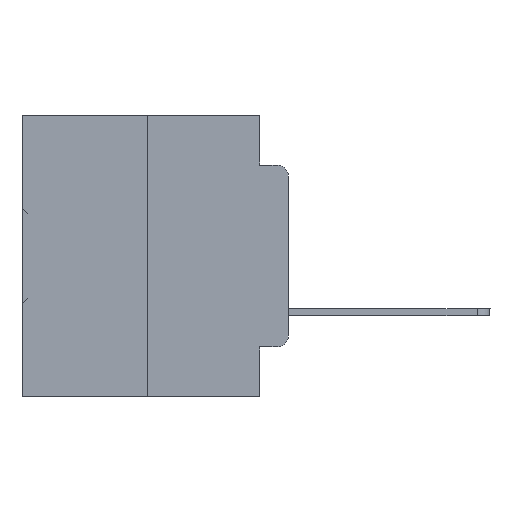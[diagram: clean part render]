
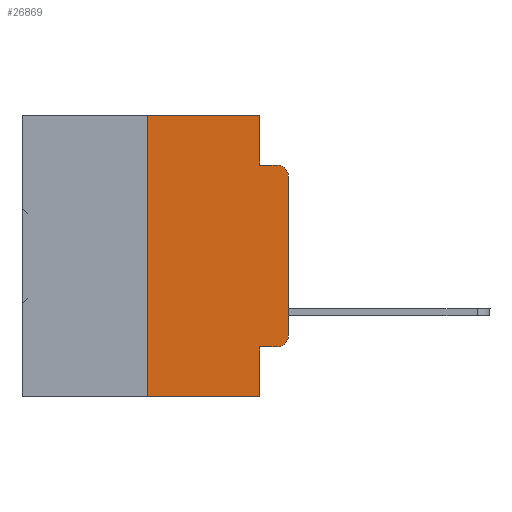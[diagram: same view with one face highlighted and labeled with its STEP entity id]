
A CAD part, left-side view. The second image highlights one B-rep face of the part: STEP entity #26869.
In plain terms, the highlighted planar face has unit normal (-1, 0, 0).
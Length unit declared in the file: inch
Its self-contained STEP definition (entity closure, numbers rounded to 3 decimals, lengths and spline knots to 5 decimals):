
#126 = VERTEX_POINT ( 'NONE', #30099 ) ;
#490 = LINE ( 'NONE', #19398, #20728 ) ;
#538 = ORIENTED_EDGE ( 'NONE', *, *, #15518, .T. ) ;
#1044 = VERTEX_POINT ( 'NONE', #1634 ) ;
#1201 = CARTESIAN_POINT ( 'NONE',  ( 0., 0.473, 0. ) ) ;
#1383 = VECTOR ( 'NONE', #17921, 39.37008 ) ;
#1459 = EDGE_CURVE ( 'NONE', #26376, #28990, #25783, .T. ) ;
#1634 = CARTESIAN_POINT ( 'NONE',  ( 0., 0.051, -0.5 ) ) ;
#2122 = ORIENTED_EDGE ( 'NONE', *, *, #19905, .F. ) ;
#2358 = EDGE_CURVE ( 'NONE', #27264, #26376, #7809, .T. ) ;
#2531 = DIRECTION ( 'NONE',  ( 0., 0., -1. ) ) ;
#3385 = CARTESIAN_POINT ( 'NONE',  ( 0., 0.051, -0.4115 ) ) ;
#4069 = VECTOR ( 'NONE', #15227, 39.37008 ) ;
#5417 = ORIENTED_EDGE ( 'NONE', *, *, #25851, .T. ) ;
#5433 = CARTESIAN_POINT ( 'NONE',  ( 0., 0.02, -0.4115 ) ) ;
#5965 = EDGE_CURVE ( 'NONE', #28134, #1044, #12391, .T. ) ;
#6599 = VERTEX_POINT ( 'NONE', #24161 ) ;
#6782 = DIRECTION ( 'NONE',  ( 0., -1., 0. ) ) ;
#6869 = VERTEX_POINT ( 'NONE', #23663 ) ;
#7082 = DIRECTION ( 'NONE',  ( 0., 0., -1. ) ) ;
#7211 = CARTESIAN_POINT ( 'NONE',  ( 0., 0.473, -0.5 ) ) ;
#7809 = CIRCLE ( 'NONE', #18820, 0.02 ) ;
#7995 = CARTESIAN_POINT ( 'NONE',  ( 0., 0., -0.3915 ) ) ;
#8035 = CARTESIAN_POINT ( 'NONE',  ( 0., 0.25, -0.5 ) ) ;
#8960 = DIRECTION ( 'NONE',  ( 0., 0., -1. ) ) ;
#9674 = CARTESIAN_POINT ( 'NONE',  ( 0., 0.051, 0. ) ) ;
#9696 = CARTESIAN_POINT ( 'NONE',  ( 0., 0.051, -0.4115 ) ) ;
#9814 = LINE ( 'NONE', #20336, #25372 ) ;
#10351 = LINE ( 'NONE', #22161, #12991 ) ;
#10411 = PLANE ( 'NONE',  #27936 ) ;
#10488 = LINE ( 'NONE', #18305, #18706 ) ;
#10786 = EDGE_LOOP ( 'NONE', ( #19140, #538, #18006, #33242, #21873, #2122, #30700, #25112, #5417, #28269 ) ) ;
#10952 = VERTEX_POINT ( 'NONE', #8035 ) ;
#12114 = LINE ( 'NONE', #7211, #1383 ) ;
#12391 = LINE ( 'NONE', #9674, #32156 ) ;
#12475 = DIRECTION ( 'NONE',  ( -1., 0., 0. ) ) ;
#12529 = VERTEX_POINT ( 'NONE', #23662 ) ;
#12991 = VECTOR ( 'NONE', #30169, 39.37008 ) ;
#13649 = AXIS2_PLACEMENT_3D ( 'NONE', #26289, #12475, #15550 ) ;
#15193 = VECTOR ( 'NONE', #6782, 39.37008 ) ;
#15227 = DIRECTION ( 'NONE',  ( 0., 0., 1. ) ) ;
#15518 = EDGE_CURVE ( 'NONE', #28990, #6869, #16547, .T. ) ;
#15550 = DIRECTION ( 'NONE',  ( 0., 0., -1. ) ) ;
#16495 = DIRECTION ( 'NONE',  ( 0., 0., 1. ) ) ;
#16547 = CIRCLE ( 'NONE', #13649, 0.02 ) ;
#17921 = DIRECTION ( 'NONE',  ( 0., -1., 0. ) ) ;
#18006 = ORIENTED_EDGE ( 'NONE', *, *, #27863, .F. ) ;
#18305 = CARTESIAN_POINT ( 'NONE',  ( 0., 0.051, -0.0885 ) ) ;
#18568 = LINE ( 'NONE', #9696, #15193 ) ;
#18706 = VECTOR ( 'NONE', #20845, 39.37008 ) ;
#18820 = AXIS2_PLACEMENT_3D ( 'NONE', #24178, #35277, #2531 ) ;
#19140 = ORIENTED_EDGE ( 'NONE', *, *, #1459, .T. ) ;
#19398 = CARTESIAN_POINT ( 'NONE',  ( 0., 0.25, 0. ) ) ;
#19905 = EDGE_CURVE ( 'NONE', #10952, #126, #490, .T. ) ;
#20336 = CARTESIAN_POINT ( 'NONE',  ( 0., 0.051, 0. ) ) ;
#20728 = VECTOR ( 'NONE', #16495, 39.37008 ) ;
#20845 = DIRECTION ( 'NONE',  ( 0., -1., 0. ) ) ;
#21873 = ORIENTED_EDGE ( 'NONE', *, *, #29247, .F. ) ;
#22161 = CARTESIAN_POINT ( 'NONE',  ( 0., 0.473, 0. ) ) ;
#22381 = CARTESIAN_POINT ( 'NONE',  ( 0., 0., -0.1085 ) ) ;
#23033 = DIRECTION ( 'NONE',  ( 1., 0., 0. ) ) ;
#23662 = CARTESIAN_POINT ( 'NONE',  ( 0., 0.051, 0. ) ) ;
#23663 = CARTESIAN_POINT ( 'NONE',  ( 0., 0.02, -0.0885 ) ) ;
#24161 = CARTESIAN_POINT ( 'NONE',  ( 0., 0.051, -0.0885 ) ) ;
#24178 = CARTESIAN_POINT ( 'NONE',  ( 0., 0.02, -0.3915 ) ) ;
#25112 = ORIENTED_EDGE ( 'NONE', *, *, #5965, .F. ) ;
#25372 = VECTOR ( 'NONE', #7082, 39.37008 ) ;
#25783 = LINE ( 'NONE', #31790, #4069 ) ;
#25851 = EDGE_CURVE ( 'NONE', #28134, #27264, #18568, .T. ) ;
#26289 = CARTESIAN_POINT ( 'NONE',  ( 0., 0.02, -0.1085 ) ) ;
#26376 = VERTEX_POINT ( 'NONE', #7995 ) ;
#26869 = ADVANCED_FACE ( 'NONE', ( #31764 ), #10411, .F. ) ;
#27264 = VERTEX_POINT ( 'NONE', #5433 ) ;
#27863 = EDGE_CURVE ( 'NONE', #6599, #6869, #10488, .T. ) ;
#27936 = AXIS2_PLACEMENT_3D ( 'NONE', #1201, #23033, #32602 ) ;
#28134 = VERTEX_POINT ( 'NONE', #3385 ) ;
#28269 = ORIENTED_EDGE ( 'NONE', *, *, #2358, .T. ) ;
#28990 = VERTEX_POINT ( 'NONE', #22381 ) ;
#29247 = EDGE_CURVE ( 'NONE', #126, #12529, #10351, .T. ) ;
#30099 = CARTESIAN_POINT ( 'NONE',  ( 0., 0.25, 0. ) ) ;
#30169 = DIRECTION ( 'NONE',  ( 0., -1., 0. ) ) ;
#30700 = ORIENTED_EDGE ( 'NONE', *, *, #31389, .T. ) ;
#31389 = EDGE_CURVE ( 'NONE', #10952, #1044, #12114, .T. ) ;
#31764 = FACE_OUTER_BOUND ( 'NONE', #10786, .T. ) ;
#31790 = CARTESIAN_POINT ( 'NONE',  ( 0., 0., 0. ) ) ;
#32156 = VECTOR ( 'NONE', #8960, 39.37008 ) ;
#32602 = DIRECTION ( 'NONE',  ( 0., 0., -1. ) ) ;
#33242 = ORIENTED_EDGE ( 'NONE', *, *, #33794, .F. ) ;
#33794 = EDGE_CURVE ( 'NONE', #12529, #6599, #9814, .T. ) ;
#35277 = DIRECTION ( 'NONE',  ( -1., 0., 0. ) ) ;
